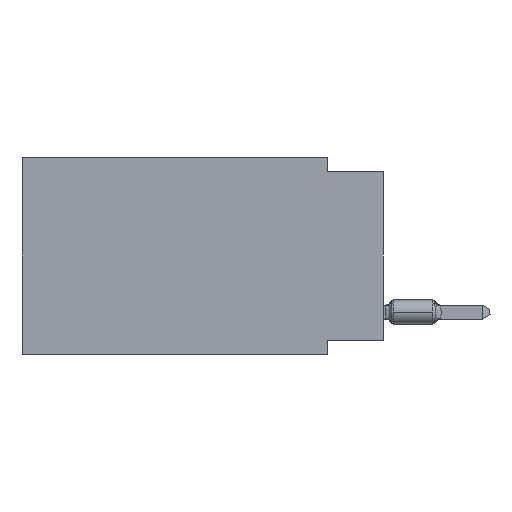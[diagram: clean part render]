
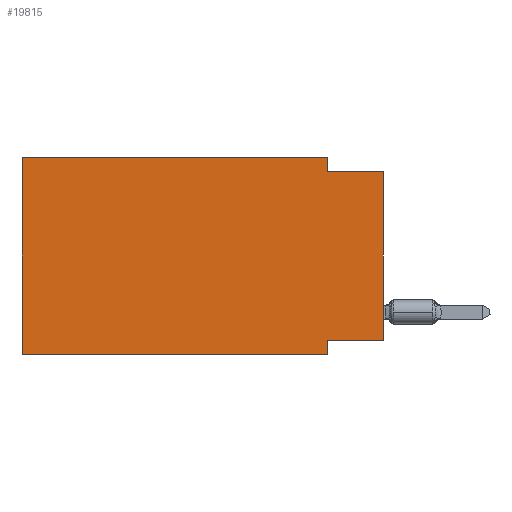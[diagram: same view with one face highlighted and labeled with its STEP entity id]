
A CAD part, left-side view. The second image highlights one B-rep face of the part: STEP entity #19815.
In plain terms, the highlighted planar face has unit normal (-1, 0, 0).
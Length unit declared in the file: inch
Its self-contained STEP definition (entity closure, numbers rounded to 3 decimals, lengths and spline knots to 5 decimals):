
#731 = VECTOR ( 'NONE', #17230, 39.37008 ) ;
#1127 = ORIENTED_EDGE ( 'NONE', *, *, #32756, .F. ) ;
#1247 = CARTESIAN_POINT ( 'NONE',  ( 0., 0., -0.025 ) ) ;
#1440 = VERTEX_POINT ( 'NONE', #30548 ) ;
#1706 = FACE_OUTER_BOUND ( 'NONE', #22296, .T. ) ;
#2077 = LINE ( 'NONE', #5127, #18093 ) ;
#2249 = VECTOR ( 'NONE', #12852, 39.37008 ) ;
#2581 = CARTESIAN_POINT ( 'NONE',  ( 0., 0.645, -0.35 ) ) ;
#2728 = DIRECTION ( 'NONE',  ( 0., 0., 1. ) ) ;
#2996 = VERTEX_POINT ( 'NONE', #1247 ) ;
#3736 = ORIENTED_EDGE ( 'NONE', *, *, #9781, .T. ) ;
#4243 = LINE ( 'NONE', #6949, #18127 ) ;
#4398 = EDGE_CURVE ( 'NONE', #5852, #20499, #23477, .T. ) ;
#4411 = DIRECTION ( 'NONE',  ( 1., 0., 0. ) ) ;
#4916 = PLANE ( 'NONE',  #25702 ) ;
#5127 = CARTESIAN_POINT ( 'NONE',  ( 0., 0.645, 0. ) ) ;
#5848 = EDGE_CURVE ( 'NONE', #19494, #2996, #28346, .T. ) ;
#5852 = VERTEX_POINT ( 'NONE', #33601 ) ;
#6560 = CARTESIAN_POINT ( 'NONE',  ( 0., 0.645, 0. ) ) ;
#6843 = CARTESIAN_POINT ( 'NONE',  ( 0., 0., -0.325 ) ) ;
#6949 = CARTESIAN_POINT ( 'NONE',  ( 0., 0., 0. ) ) ;
#9094 = ORIENTED_EDGE ( 'NONE', *, *, #9456, .F. ) ;
#9412 = VECTOR ( 'NONE', #21872, 39.37008 ) ;
#9456 = EDGE_CURVE ( 'NONE', #5852, #30630, #2077, .T. ) ;
#9781 = EDGE_CURVE ( 'NONE', #15116, #2996, #4243, .T. ) ;
#10751 = CARTESIAN_POINT ( 'NONE',  ( 0., 0.645, 0. ) ) ;
#11440 = VECTOR ( 'NONE', #23245, 39.37008 ) ;
#12852 = DIRECTION ( 'NONE',  ( 0., 0., -1. ) ) ;
#13183 = LINE ( 'NONE', #23562, #2249 ) ;
#13249 = CARTESIAN_POINT ( 'NONE',  ( 0., 0.1, -0.35 ) ) ;
#13336 = EDGE_CURVE ( 'NONE', #15116, #13631, #28239, .T. ) ;
#13631 = VERTEX_POINT ( 'NONE', #25953 ) ;
#14131 = ORIENTED_EDGE ( 'NONE', *, *, #4398, .T. ) ;
#14850 = ORIENTED_EDGE ( 'NONE', *, *, #5848, .F. ) ;
#15116 = VERTEX_POINT ( 'NONE', #27857 ) ;
#15452 = CARTESIAN_POINT ( 'NONE',  ( 0., 0., -0.025 ) ) ;
#15953 = VECTOR ( 'NONE', #31445, 39.37008 ) ;
#17116 = EDGE_CURVE ( 'NONE', #13631, #20499, #26795, .T. ) ;
#17230 = DIRECTION ( 'NONE',  ( 0., 1., 0. ) ) ;
#18093 = VECTOR ( 'NONE', #2728, 39.37008 ) ;
#18127 = VECTOR ( 'NONE', #30230, 39.37008 ) ;
#19494 = VERTEX_POINT ( 'NONE', #30942 ) ;
#19815 = ADVANCED_FACE ( 'NONE', ( #1706 ), #4916, .F. ) ;
#20051 = CARTESIAN_POINT ( 'NONE',  ( 0., 0.645, 0. ) ) ;
#20499 = VERTEX_POINT ( 'NONE', #24166 ) ;
#21449 = EDGE_CURVE ( 'NONE', #30630, #1440, #30014, .T. ) ;
#21513 = DIRECTION ( 'NONE',  ( 0., 0., -1. ) ) ;
#21872 = DIRECTION ( 'NONE',  ( 0., -1., 0. ) ) ;
#22296 = EDGE_LOOP ( 'NONE', ( #3736, #14850, #1127, #27311, #9094, #14131, #32356, #25227 ) ) ;
#23245 = DIRECTION ( 'NONE',  ( 0., -1., 0. ) ) ;
#23477 = LINE ( 'NONE', #2581, #15953 ) ;
#23562 = CARTESIAN_POINT ( 'NONE',  ( 0., 0.1, 0. ) ) ;
#24166 = CARTESIAN_POINT ( 'NONE',  ( 0., 0.1, -0.35 ) ) ;
#25227 = ORIENTED_EDGE ( 'NONE', *, *, #13336, .F. ) ;
#25702 = AXIS2_PLACEMENT_3D ( 'NONE', #20051, #4411, #30748 ) ;
#25953 = CARTESIAN_POINT ( 'NONE',  ( 0., 0.1, -0.325 ) ) ;
#26795 = LINE ( 'NONE', #13249, #29778 ) ;
#27311 = ORIENTED_EDGE ( 'NONE', *, *, #21449, .F. ) ;
#27857 = CARTESIAN_POINT ( 'NONE',  ( 0., 0., -0.325 ) ) ;
#28239 = LINE ( 'NONE', #6843, #731 ) ;
#28346 = LINE ( 'NONE', #15452, #11440 ) ;
#29778 = VECTOR ( 'NONE', #21513, 39.37008 ) ;
#30014 = LINE ( 'NONE', #6560, #9412 ) ;
#30230 = DIRECTION ( 'NONE',  ( 0., 0., 1. ) ) ;
#30548 = CARTESIAN_POINT ( 'NONE',  ( 0., 0.1, 0. ) ) ;
#30630 = VERTEX_POINT ( 'NONE', #10751 ) ;
#30748 = DIRECTION ( 'NONE',  ( 0., 0., -1. ) ) ;
#30942 = CARTESIAN_POINT ( 'NONE',  ( 0., 0.1, -0.025 ) ) ;
#31445 = DIRECTION ( 'NONE',  ( 0., -1., 0. ) ) ;
#32356 = ORIENTED_EDGE ( 'NONE', *, *, #17116, .F. ) ;
#32756 = EDGE_CURVE ( 'NONE', #1440, #19494, #13183, .T. ) ;
#33601 = CARTESIAN_POINT ( 'NONE',  ( 0., 0.645, -0.35 ) ) ;
